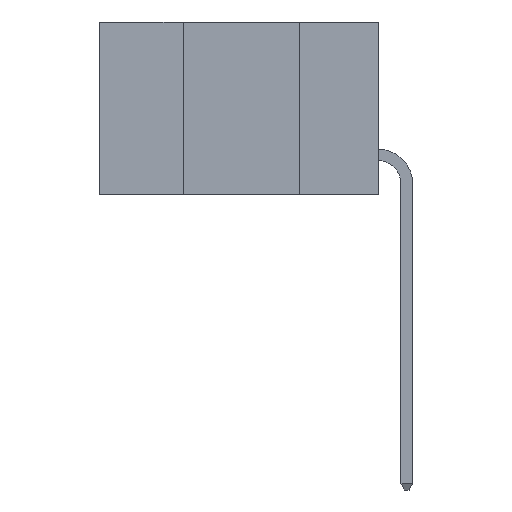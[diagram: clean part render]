
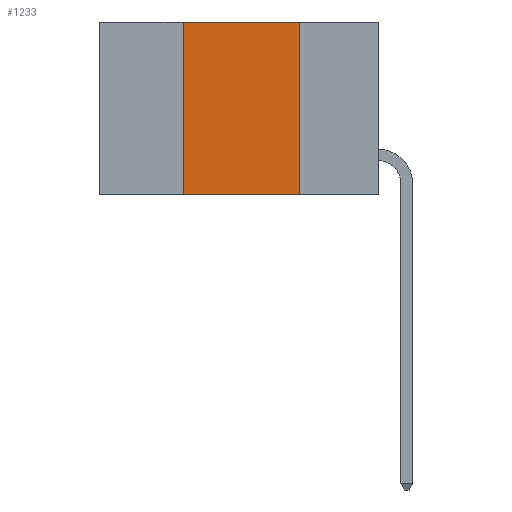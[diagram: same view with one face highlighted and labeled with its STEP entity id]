
A CAD part, left-side view. The second image highlights one B-rep face of the part: STEP entity #1233.
In plain terms, the highlighted planar face has unit normal (-1, 0, 0).
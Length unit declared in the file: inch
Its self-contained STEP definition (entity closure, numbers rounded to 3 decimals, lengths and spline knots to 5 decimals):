
#81 = EDGE_CURVE ( 'NONE', #3763, #5729, #456, .T. ) ;
#244 = EDGE_CURVE ( 'NONE', #11628, #13539, #13487, .T. ) ;
#456 = LINE ( 'NONE', #2792, #2206 ) ;
#1233 = ADVANCED_FACE ( 'NONE', ( #11196 ), #7043, .F. ) ;
#1505 = DIRECTION ( 'NONE',  ( 0., -1., 0. ) ) ;
#1512 = CARTESIAN_POINT ( 'NONE',  ( 0., 0.17, -0.37 ) ) ;
#2206 = VECTOR ( 'NONE', #9343, 39.37008 ) ;
#2321 = VECTOR ( 'NONE', #1505, 39.37008 ) ;
#2792 = CARTESIAN_POINT ( 'NONE',  ( 0., 0.42, -0.37 ) ) ;
#3763 = VERTEX_POINT ( 'NONE', #10923 ) ;
#4251 = ORIENTED_EDGE ( 'NONE', *, *, #81, .F. ) ;
#4335 = DIRECTION ( 'NONE',  ( 0., -1., 0. ) ) ;
#4426 = LINE ( 'NONE', #6989, #2321 ) ;
#5455 = ORIENTED_EDGE ( 'NONE', *, *, #244, .F. ) ;
#5729 = VERTEX_POINT ( 'NONE', #10561 ) ;
#5885 = CARTESIAN_POINT ( 'NONE',  ( 0., 0.6, 0. ) ) ;
#6989 = CARTESIAN_POINT ( 'NONE',  ( 0., 0.6, 0. ) ) ;
#6994 = DIRECTION ( 'NONE',  ( 0., 0., -1. ) ) ;
#7043 = PLANE ( 'NONE',  #13780 ) ;
#7333 = LINE ( 'NONE', #11902, #10982 ) ;
#7605 = ORIENTED_EDGE ( 'NONE', *, *, #8948, .F. ) ;
#7905 = VECTOR ( 'NONE', #8076, 39.37008 ) ;
#8076 = DIRECTION ( 'NONE',  ( 0., 0., -1. ) ) ;
#8461 = ORIENTED_EDGE ( 'NONE', *, *, #11070, .T. ) ;
#8548 = CARTESIAN_POINT ( 'NONE',  ( 0., 0.17, 0. ) ) ;
#8948 = EDGE_CURVE ( 'NONE', #5729, #11628, #4426, .T. ) ;
#9343 = DIRECTION ( 'NONE',  ( 0., 0., 1. ) ) ;
#10561 = CARTESIAN_POINT ( 'NONE',  ( 0., 0.42, 0. ) ) ;
#10923 = CARTESIAN_POINT ( 'NONE',  ( 0., 0.42, -0.37 ) ) ;
#10982 = VECTOR ( 'NONE', #4335, 39.37008 ) ;
#11070 = EDGE_CURVE ( 'NONE', #3763, #13539, #7333, .T. ) ;
#11196 = FACE_OUTER_BOUND ( 'NONE', #13246, .T. ) ;
#11305 = CARTESIAN_POINT ( 'NONE',  ( 0., 0.17, -0.37 ) ) ;
#11426 = DIRECTION ( 'NONE',  ( 1., 0., 0. ) ) ;
#11628 = VERTEX_POINT ( 'NONE', #8548 ) ;
#11902 = CARTESIAN_POINT ( 'NONE',  ( 0., 0.6, -0.37 ) ) ;
#13246 = EDGE_LOOP ( 'NONE', ( #5455, #7605, #4251, #8461 ) ) ;
#13487 = LINE ( 'NONE', #11305, #7905 ) ;
#13539 = VERTEX_POINT ( 'NONE', #1512 ) ;
#13780 = AXIS2_PLACEMENT_3D ( 'NONE', #5885, #11426, #6994 ) ;
